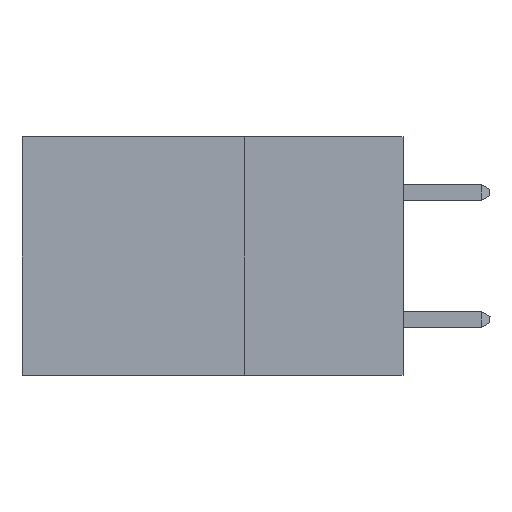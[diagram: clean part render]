
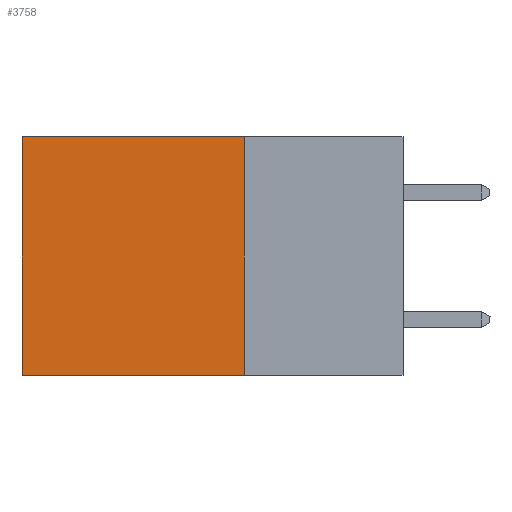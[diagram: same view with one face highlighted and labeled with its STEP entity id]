
A CAD part, left-side view. The second image highlights one B-rep face of the part: STEP entity #3758.
In plain terms, the highlighted planar face has unit normal (-1, 0, 0).
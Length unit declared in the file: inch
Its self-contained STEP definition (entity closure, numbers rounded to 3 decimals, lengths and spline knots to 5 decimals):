
#1019 = FACE_OUTER_BOUND ( 'NONE', #1766, .T. ) ;
#1766 = EDGE_LOOP ( 'NONE', ( #6722, #12417, #16504, #15686 ) ) ;
#1774 = DIRECTION ( 'NONE',  ( 0., 0., -1. ) ) ;
#2416 = CARTESIAN_POINT ( 'NONE',  ( 0.2875, 0.6, -0.375 ) ) ;
#2992 = VECTOR ( 'NONE', #4216, 39.37008 ) ;
#3232 = DIRECTION ( 'NONE',  ( 1., 0., 0. ) ) ;
#3758 = ADVANCED_FACE ( 'NONE', ( #1019 ), #5633, .F. ) ;
#4216 = DIRECTION ( 'NONE',  ( 0., 1., 0. ) ) ;
#4231 = CARTESIAN_POINT ( 'NONE',  ( 0.2875, 0.25, 0. ) ) ;
#4377 = CARTESIAN_POINT ( 'NONE',  ( 0.2875, 0.6, -0.375 ) ) ;
#5279 = LINE ( 'NONE', #17492, #2992 ) ;
#5333 = VERTEX_POINT ( 'NONE', #2416 ) ;
#5453 = VECTOR ( 'NONE', #14602, 39.37008 ) ;
#5633 = PLANE ( 'NONE',  #6550 ) ;
#6061 = VECTOR ( 'NONE', #12707, 39.37008 ) ;
#6139 = CARTESIAN_POINT ( 'NONE',  ( 0.2875, 0.25, -0.375 ) ) ;
#6550 = AXIS2_PLACEMENT_3D ( 'NONE', #9307, #3232, #13663 ) ;
#6653 = EDGE_CURVE ( 'NONE', #8609, #5333, #5279, .T. ) ;
#6722 = ORIENTED_EDGE ( 'NONE', *, *, #16809, .T. ) ;
#7486 = CARTESIAN_POINT ( 'NONE',  ( 0.2875, 0.6, 0. ) ) ;
#7574 = VECTOR ( 'NONE', #1774, 39.37008 ) ;
#8609 = VERTEX_POINT ( 'NONE', #16924 ) ;
#9307 = CARTESIAN_POINT ( 'NONE',  ( 0.2875, 0.25, -0.375 ) ) ;
#9698 = VERTEX_POINT ( 'NONE', #7486 ) ;
#10100 = EDGE_CURVE ( 'NONE', #15201, #9698, #10859, .T. ) ;
#10859 = LINE ( 'NONE', #4231, #6061 ) ;
#11424 = LINE ( 'NONE', #6139, #7574 ) ;
#12417 = ORIENTED_EDGE ( 'NONE', *, *, #6653, .F. ) ;
#12707 = DIRECTION ( 'NONE',  ( 0., 1., 0. ) ) ;
#13663 = DIRECTION ( 'NONE',  ( 0., 0., -1. ) ) ;
#14357 = CARTESIAN_POINT ( 'NONE',  ( 0.2875, 0.25, 0. ) ) ;
#14602 = DIRECTION ( 'NONE',  ( 0., 0., -1. ) ) ;
#15070 = LINE ( 'NONE', #4377, #5453 ) ;
#15201 = VERTEX_POINT ( 'NONE', #14357 ) ;
#15686 = ORIENTED_EDGE ( 'NONE', *, *, #10100, .T. ) ;
#16231 = EDGE_CURVE ( 'NONE', #15201, #8609, #11424, .T. ) ;
#16504 = ORIENTED_EDGE ( 'NONE', *, *, #16231, .F. ) ;
#16809 = EDGE_CURVE ( 'NONE', #9698, #5333, #15070, .T. ) ;
#16924 = CARTESIAN_POINT ( 'NONE',  ( 0.2875, 0.25, -0.375 ) ) ;
#17492 = CARTESIAN_POINT ( 'NONE',  ( 0.2875, 0.25, -0.375 ) ) ;
